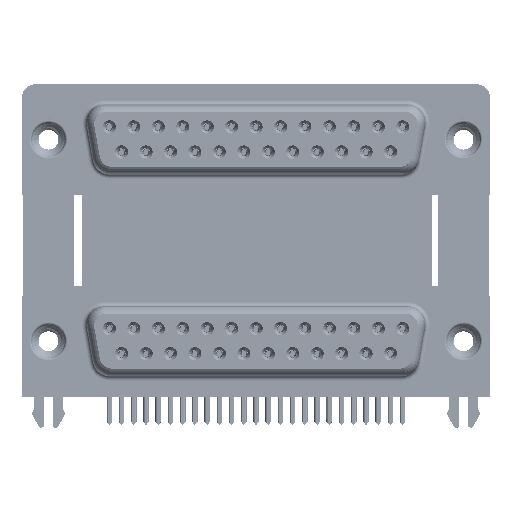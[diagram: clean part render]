
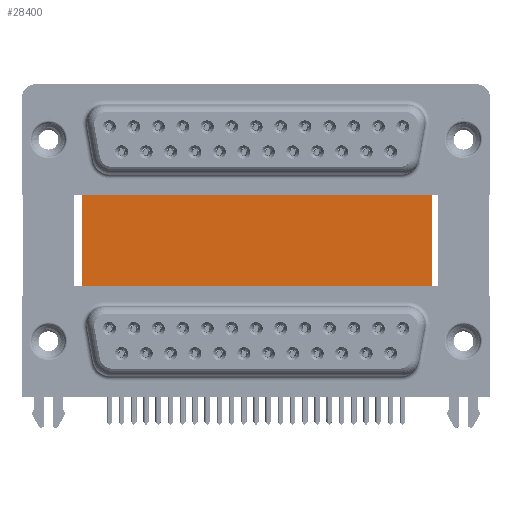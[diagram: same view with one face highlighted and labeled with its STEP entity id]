
A CAD part, top view. The second image highlights one B-rep face of the part: STEP entity #28400.
In plain terms, the highlighted planar face has unit normal (0, 0, 1).
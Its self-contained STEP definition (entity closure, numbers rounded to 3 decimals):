
#988 = DIRECTION ( 'NONE',  ( 0., 0., -1. ) ) ;
#1589 = CARTESIAN_POINT ( 'NONE',  ( 3.79, 16.585, -12. ) ) ;
#1841 = ORIENTED_EDGE ( 'NONE', *, *, #30833, .T. ) ;
#12439 = CARTESIAN_POINT ( 'NONE',  ( 3.79, 16.585, -12. ) ) ;
#12612 = CARTESIAN_POINT ( 'NONE',  ( 43.43, 16.585, -12. ) ) ;
#13731 = LINE ( 'NONE', #61346, #61533 ) ;
#15510 = DIRECTION ( 'NONE',  ( -1., 0., 0. ) ) ;
#15883 = VERTEX_POINT ( 'NONE', #21085 ) ;
#17026 = CARTESIAN_POINT ( 'NONE',  ( 3.79, -3.735, -12. ) ) ;
#17078 = ORIENTED_EDGE ( 'NONE', *, *, #55353, .F. ) ;
#20202 = ORIENTED_EDGE ( 'NONE', *, *, #20639, .T. ) ;
#20271 = FACE_OUTER_BOUND ( 'NONE', #33737, .T. ) ;
#20639 = EDGE_CURVE ( 'NONE', #26093, #53951, #41316, .T. ) ;
#21085 = CARTESIAN_POINT ( 'NONE',  ( 43.43, -3.735, -12. ) ) ;
#21744 = VECTOR ( 'NONE', #51446, 1000. ) ;
#26093 = VERTEX_POINT ( 'NONE', #12439 ) ;
#27253 = CARTESIAN_POINT ( 'NONE',  ( 43.43, 16.585, -12. ) ) ;
#27347 = ORIENTED_EDGE ( 'NONE', *, *, #45610, .F. ) ;
#27868 = LINE ( 'NONE', #27253, #21744 ) ;
#28400 = ADVANCED_FACE ( 'NONE', ( #20271 ), #34122, .F. ) ;
#30365 = CARTESIAN_POINT ( 'NONE',  ( 3.79, -3.735, -12. ) ) ;
#30833 = EDGE_CURVE ( 'NONE', #53951, #15883, #58390, .T. ) ;
#33737 = EDGE_LOOP ( 'NONE', ( #1841, #27347, #17078, #20202 ) ) ;
#34122 = PLANE ( 'NONE',  #57944 ) ;
#36879 = CARTESIAN_POINT ( 'NONE',  ( 3.79, 16.585, -12. ) ) ;
#38162 = VERTEX_POINT ( 'NONE', #12612 ) ;
#39190 = DIRECTION ( 'NONE',  ( 1., 0., 0. ) ) ;
#41316 = LINE ( 'NONE', #36879, #50536 ) ;
#45610 = EDGE_CURVE ( 'NONE', #38162, #15883, #27868, .T. ) ;
#50536 = VECTOR ( 'NONE', #60522, 1000. ) ;
#51446 = DIRECTION ( 'NONE',  ( 0., -1., 0. ) ) ;
#53951 = VERTEX_POINT ( 'NONE', #17026 ) ;
#55353 = EDGE_CURVE ( 'NONE', #26093, #38162, #13731, .T. ) ;
#55672 = DIRECTION ( 'NONE',  ( 1., 0., 0. ) ) ;
#56128 = VECTOR ( 'NONE', #39190, 1000. ) ;
#57944 = AXIS2_PLACEMENT_3D ( 'NONE', #1589, #988, #15510 ) ;
#58390 = LINE ( 'NONE', #30365, #56128 ) ;
#60522 = DIRECTION ( 'NONE',  ( 0., -1., 0. ) ) ;
#61346 = CARTESIAN_POINT ( 'NONE',  ( 3.79, 16.585, -12. ) ) ;
#61533 = VECTOR ( 'NONE', #55672, 1000. ) ;
